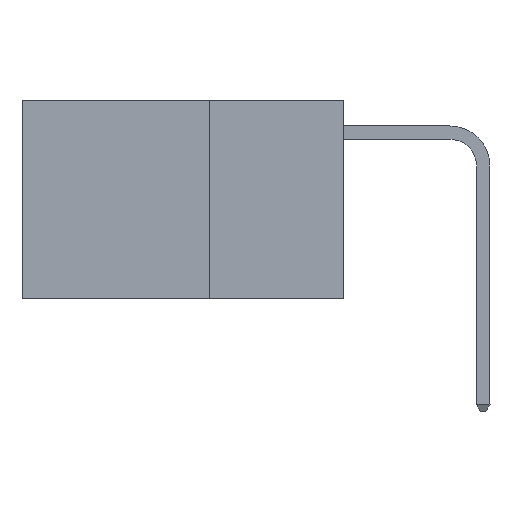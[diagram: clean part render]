
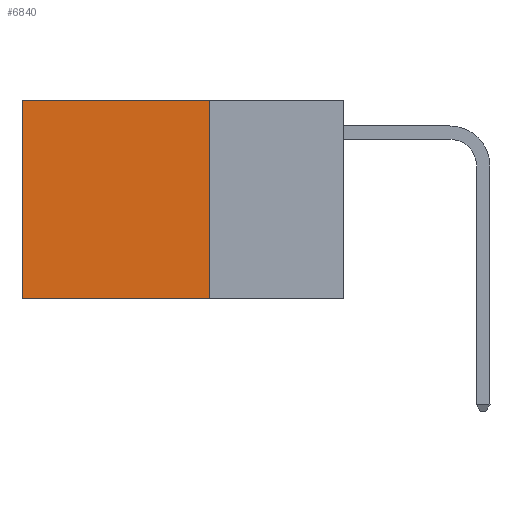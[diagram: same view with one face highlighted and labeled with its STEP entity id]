
A CAD part, left-side view. The second image highlights one B-rep face of the part: STEP entity #6840.
In plain terms, the highlighted planar face has unit normal (-1, 0, 0).
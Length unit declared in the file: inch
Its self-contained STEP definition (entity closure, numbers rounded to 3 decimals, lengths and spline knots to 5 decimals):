
#56 = EDGE_CURVE ( 'NONE', #10266, #4631, #8630, .T. ) ;
#118 = DIRECTION ( 'NONE',  ( 0., 1., 0. ) ) ;
#326 = LINE ( 'NONE', #6514, #10232 ) ;
#855 = CARTESIAN_POINT ( 'NONE',  ( 0.2625, 0.25, 0. ) ) ;
#969 = CARTESIAN_POINT ( 'NONE',  ( 0.2625, 0.25, 0. ) ) ;
#1954 = DIRECTION ( 'NONE',  ( 0., 0., -1. ) ) ;
#2625 = VERTEX_POINT ( 'NONE', #13187 ) ;
#2741 = LINE ( 'NONE', #969, #10388 ) ;
#3169 = DIRECTION ( 'NONE',  ( 0., 1., 0. ) ) ;
#3208 = VERTEX_POINT ( 'NONE', #5697 ) ;
#3651 = LINE ( 'NONE', #4147, #11513 ) ;
#4147 = CARTESIAN_POINT ( 'NONE',  ( 0.2625, 0.25, 0. ) ) ;
#4154 = CARTESIAN_POINT ( 'NONE',  ( 0.2625, 0.25, -0.37 ) ) ;
#4323 = DIRECTION ( 'NONE',  ( 0., 0., -1. ) ) ;
#4565 = EDGE_LOOP ( 'NONE', ( #6687, #7219, #7695, #7558 ) ) ;
#4631 = VERTEX_POINT ( 'NONE', #9542 ) ;
#4766 = FACE_OUTER_BOUND ( 'NONE', #4565, .T. ) ;
#5124 = EDGE_CURVE ( 'NONE', #2625, #10266, #3651, .T. ) ;
#5697 = CARTESIAN_POINT ( 'NONE',  ( 0.2625, 0.6, 0. ) ) ;
#5925 = VECTOR ( 'NONE', #118, 39.37008 ) ;
#6477 = DIRECTION ( 'NONE',  ( 0., 0., -1. ) ) ;
#6514 = CARTESIAN_POINT ( 'NONE',  ( 0.2625, 0.6, 0. ) ) ;
#6687 = ORIENTED_EDGE ( 'NONE', *, *, #12667, .T. ) ;
#6840 = ADVANCED_FACE ( 'NONE', ( #4766 ), #12218, .F. ) ;
#7219 = ORIENTED_EDGE ( 'NONE', *, *, #56, .F. ) ;
#7558 = ORIENTED_EDGE ( 'NONE', *, *, #11957, .T. ) ;
#7695 = ORIENTED_EDGE ( 'NONE', *, *, #5124, .F. ) ;
#8084 = CARTESIAN_POINT ( 'NONE',  ( 0.2625, 0.25, -0.37 ) ) ;
#8395 = DIRECTION ( 'NONE',  ( 1., 0., 0. ) ) ;
#8630 = LINE ( 'NONE', #4154, #5925 ) ;
#9326 = AXIS2_PLACEMENT_3D ( 'NONE', #855, #8395, #1954 ) ;
#9542 = CARTESIAN_POINT ( 'NONE',  ( 0.2625, 0.6, -0.37 ) ) ;
#10232 = VECTOR ( 'NONE', #6477, 39.37008 ) ;
#10266 = VERTEX_POINT ( 'NONE', #8084 ) ;
#10388 = VECTOR ( 'NONE', #3169, 39.37008 ) ;
#11513 = VECTOR ( 'NONE', #4323, 39.37008 ) ;
#11957 = EDGE_CURVE ( 'NONE', #2625, #3208, #2741, .T. ) ;
#12218 = PLANE ( 'NONE',  #9326 ) ;
#12667 = EDGE_CURVE ( 'NONE', #3208, #4631, #326, .T. ) ;
#13187 = CARTESIAN_POINT ( 'NONE',  ( 0.2625, 0.25, 0. ) ) ;
